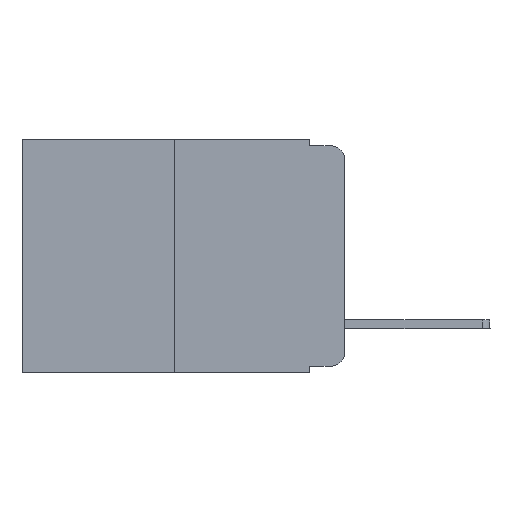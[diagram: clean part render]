
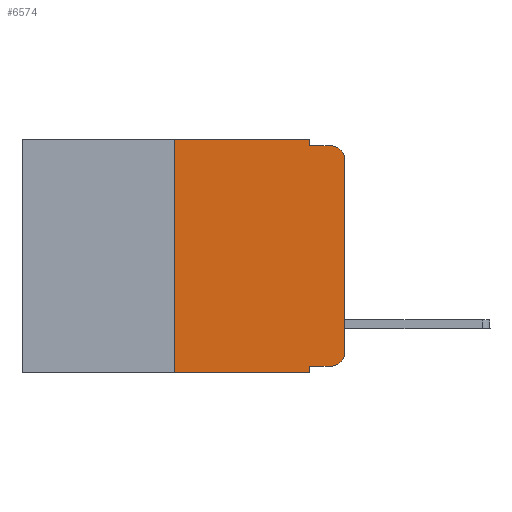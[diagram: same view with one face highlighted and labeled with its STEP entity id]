
A CAD part, left-side view. The second image highlights one B-rep face of the part: STEP entity #6574.
In plain terms, the highlighted planar face has unit normal (-1, 0, 0).
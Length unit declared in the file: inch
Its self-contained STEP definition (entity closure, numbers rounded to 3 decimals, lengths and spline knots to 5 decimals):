
#139 = DIRECTION ( 'NONE',  ( 0., 0., -1. ) ) ;
#208 = ORIENTED_EDGE ( 'NONE', *, *, #1309, .F. ) ;
#649 = VERTEX_POINT ( 'NONE', #18817 ) ;
#785 = VERTEX_POINT ( 'NONE', #13714 ) ;
#1309 = EDGE_CURVE ( 'NONE', #649, #9638, #22875, .T. ) ;
#1674 = ORIENTED_EDGE ( 'NONE', *, *, #16637, .F. ) ;
#1865 = ORIENTED_EDGE ( 'NONE', *, *, #16305, .T. ) ;
#2144 = CARTESIAN_POINT ( 'NONE',  ( 0., 0.02, -0.03 ) ) ;
#2156 = CARTESIAN_POINT ( 'NONE',  ( 0., 0.25, -0.343 ) ) ;
#3282 = ORIENTED_EDGE ( 'NONE', *, *, #22014, .T. ) ;
#3508 = VERTEX_POINT ( 'NONE', #23113 ) ;
#3788 = CARTESIAN_POINT ( 'NONE',  ( 0., 0.02, -0.313 ) ) ;
#3916 = CARTESIAN_POINT ( 'NONE',  ( 0., 0., -0.03 ) ) ;
#4152 = CARTESIAN_POINT ( 'NONE',  ( 0., 0.051, 0. ) ) ;
#4402 = CARTESIAN_POINT ( 'NONE',  ( 0., 0.25, 0. ) ) ;
#4489 = EDGE_CURVE ( 'NONE', #11636, #9638, #6834, .T. ) ;
#4646 = LINE ( 'NONE', #21213, #14532 ) ;
#4799 = FACE_OUTER_BOUND ( 'NONE', #15076, .T. ) ;
#6243 = LINE ( 'NONE', #14459, #20161 ) ;
#6258 = LINE ( 'NONE', #10428, #14171 ) ;
#6316 = DIRECTION ( 'NONE',  ( 0., 0., 1. ) ) ;
#6574 = ADVANCED_FACE ( 'NONE', ( #4799 ), #19443, .F. ) ;
#6834 = LINE ( 'NONE', #10206, #18461 ) ;
#6840 = LINE ( 'NONE', #22989, #13592 ) ;
#7622 = ORIENTED_EDGE ( 'NONE', *, *, #10651, .F. ) ;
#8236 = EDGE_CURVE ( 'NONE', #3508, #14012, #14302, .T. ) ;
#8615 = DIRECTION ( 'NONE',  ( 0., -1., 0. ) ) ;
#8856 = DIRECTION ( 'NONE',  ( 0., -1., 0. ) ) ;
#9132 = DIRECTION ( 'NONE',  ( -1., 0., 0. ) ) ;
#9359 = CARTESIAN_POINT ( 'NONE',  ( 0., 0.051, -0.343 ) ) ;
#9381 = DIRECTION ( 'NONE',  ( -1., 0., 0. ) ) ;
#9538 = AXIS2_PLACEMENT_3D ( 'NONE', #19204, #19360, #10137 ) ;
#9638 = VERTEX_POINT ( 'NONE', #9359 ) ;
#10090 = VERTEX_POINT ( 'NONE', #11147 ) ;
#10137 = DIRECTION ( 'NONE',  ( 0., 0., -1. ) ) ;
#10206 = CARTESIAN_POINT ( 'NONE',  ( 0., 0.473, -0.343 ) ) ;
#10428 = CARTESIAN_POINT ( 'NONE',  ( 0., 0.051, -0.333 ) ) ;
#10499 = LINE ( 'NONE', #23129, #14751 ) ;
#10502 = ORIENTED_EDGE ( 'NONE', *, *, #11521, .T. ) ;
#10651 = EDGE_CURVE ( 'NONE', #15774, #785, #6840, .T. ) ;
#11073 = ORIENTED_EDGE ( 'NONE', *, *, #19479, .F. ) ;
#11147 = CARTESIAN_POINT ( 'NONE',  ( 0., 0.25, 0. ) ) ;
#11521 = EDGE_CURVE ( 'NONE', #649, #3508, #6258, .T. ) ;
#11636 = VERTEX_POINT ( 'NONE', #2156 ) ;
#13154 = DIRECTION ( 'NONE',  ( 0., 0., 1. ) ) ;
#13235 = AXIS2_PLACEMENT_3D ( 'NONE', #3788, #9132, #21552 ) ;
#13359 = ORIENTED_EDGE ( 'NONE', *, *, #4489, .T. ) ;
#13592 = VECTOR ( 'NONE', #8615, 39.37008 ) ;
#13714 = CARTESIAN_POINT ( 'NONE',  ( 0., 0.02, -0.01 ) ) ;
#13819 = VERTEX_POINT ( 'NONE', #3916 ) ;
#14012 = VERTEX_POINT ( 'NONE', #22725 ) ;
#14171 = VECTOR ( 'NONE', #8856, 39.37008 ) ;
#14302 = CIRCLE ( 'NONE', #13235, 0.02 ) ;
#14459 = CARTESIAN_POINT ( 'NONE',  ( 0., 0.051, 0. ) ) ;
#14532 = VECTOR ( 'NONE', #22864, 39.37008 ) ;
#14751 = VECTOR ( 'NONE', #6316, 39.37008 ) ;
#14955 = AXIS2_PLACEMENT_3D ( 'NONE', #2144, #9381, #20125 ) ;
#14971 = DIRECTION ( 'NONE',  ( 0., 0., -1. ) ) ;
#15076 = EDGE_LOOP ( 'NONE', ( #1865, #3282, #7622, #1674, #11073, #18999, #13359, #208, #10502, #21516 ) ) ;
#15774 = VERTEX_POINT ( 'NONE', #22909 ) ;
#16305 = EDGE_CURVE ( 'NONE', #14012, #13819, #10499, .T. ) ;
#16637 = EDGE_CURVE ( 'NONE', #17216, #15774, #6243, .T. ) ;
#16697 = CIRCLE ( 'NONE', #14955, 0.02 ) ;
#17211 = DIRECTION ( 'NONE',  ( 0., -1., 0. ) ) ;
#17216 = VERTEX_POINT ( 'NONE', #18329 ) ;
#18329 = CARTESIAN_POINT ( 'NONE',  ( 0., 0.051, 0. ) ) ;
#18461 = VECTOR ( 'NONE', #17211, 39.37008 ) ;
#18650 = VECTOR ( 'NONE', #13154, 39.37008 ) ;
#18817 = CARTESIAN_POINT ( 'NONE',  ( 0., 0.051, -0.333 ) ) ;
#18999 = ORIENTED_EDGE ( 'NONE', *, *, #22730, .F. ) ;
#19204 = CARTESIAN_POINT ( 'NONE',  ( 0., 0.473, 0. ) ) ;
#19360 = DIRECTION ( 'NONE',  ( 1., 0., 0. ) ) ;
#19443 = PLANE ( 'NONE',  #9538 ) ;
#19479 = EDGE_CURVE ( 'NONE', #10090, #17216, #4646, .T. ) ;
#20050 = VECTOR ( 'NONE', #14971, 39.37008 ) ;
#20125 = DIRECTION ( 'NONE',  ( 0., 0., -1. ) ) ;
#20161 = VECTOR ( 'NONE', #139, 39.37008 ) ;
#20376 = LINE ( 'NONE', #4402, #18650 ) ;
#21213 = CARTESIAN_POINT ( 'NONE',  ( 0., 0.473, 0. ) ) ;
#21516 = ORIENTED_EDGE ( 'NONE', *, *, #8236, .T. ) ;
#21552 = DIRECTION ( 'NONE',  ( 0., 0., -1. ) ) ;
#22014 = EDGE_CURVE ( 'NONE', #13819, #785, #16697, .T. ) ;
#22725 = CARTESIAN_POINT ( 'NONE',  ( 0., 0., -0.313 ) ) ;
#22730 = EDGE_CURVE ( 'NONE', #11636, #10090, #20376, .T. ) ;
#22864 = DIRECTION ( 'NONE',  ( 0., -1., 0. ) ) ;
#22875 = LINE ( 'NONE', #4152, #20050 ) ;
#22909 = CARTESIAN_POINT ( 'NONE',  ( 0., 0.051, -0.01 ) ) ;
#22989 = CARTESIAN_POINT ( 'NONE',  ( 0., 0.051, -0.01 ) ) ;
#23113 = CARTESIAN_POINT ( 'NONE',  ( 0., 0.02, -0.333 ) ) ;
#23129 = CARTESIAN_POINT ( 'NONE',  ( 0., 0., 0. ) ) ;
